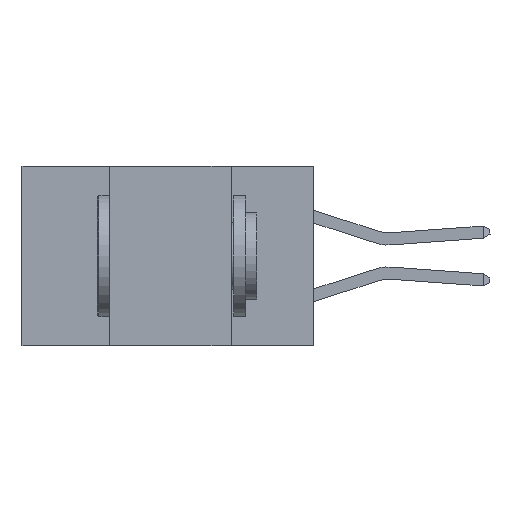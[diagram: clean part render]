
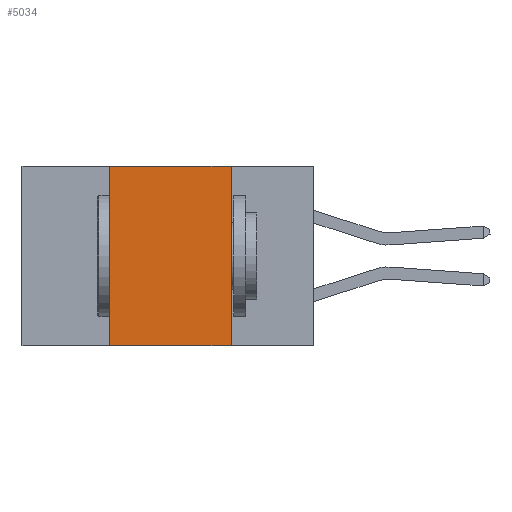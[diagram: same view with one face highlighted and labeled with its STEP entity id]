
A CAD part, left-side view. The second image highlights one B-rep face of the part: STEP entity #5034.
In plain terms, the highlighted planar face has unit normal (-1, 0, 0).
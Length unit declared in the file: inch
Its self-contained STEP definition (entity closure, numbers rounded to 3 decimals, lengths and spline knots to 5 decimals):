
#1138 = CARTESIAN_POINT ( 'NONE',  ( 0., 0.6, -0.37 ) ) ;
#3167 = VECTOR ( 'NONE', #13294, 39.37008 ) ;
#3473 = DIRECTION ( 'NONE',  ( 0., 0., -1. ) ) ;
#4010 = FACE_OUTER_BOUND ( 'NONE', #34146, .T. ) ;
#5034 = ADVANCED_FACE ( 'NONE', ( #4010 ), #29810, .F. ) ;
#6019 = ORIENTED_EDGE ( 'NONE', *, *, #39472, .F. ) ;
#6518 = AXIS2_PLACEMENT_3D ( 'NONE', #7168, #36558, #3473 ) ;
#7168 = CARTESIAN_POINT ( 'NONE',  ( 0., 0.6, 0. ) ) ;
#8007 = CARTESIAN_POINT ( 'NONE',  ( 0., 0.42, 0. ) ) ;
#8116 = VERTEX_POINT ( 'NONE', #30020 ) ;
#9017 = LINE ( 'NONE', #1138, #24797 ) ;
#9627 = LINE ( 'NONE', #25424, #29966 ) ;
#12751 = EDGE_CURVE ( 'NONE', #40426, #8116, #9017, .T. ) ;
#13294 = DIRECTION ( 'NONE',  ( 0., 0., -1. ) ) ;
#13712 = DIRECTION ( 'NONE',  ( 0., -1., 0. ) ) ;
#14030 = CARTESIAN_POINT ( 'NONE',  ( 0., 0.42, -0.37 ) ) ;
#14700 = EDGE_CURVE ( 'NONE', #40426, #26995, #36577, .T. ) ;
#17215 = VECTOR ( 'NONE', #24642, 39.37008 ) ;
#22458 = CARTESIAN_POINT ( 'NONE',  ( 0., 0.17, 0. ) ) ;
#24642 = DIRECTION ( 'NONE',  ( 0., 0., 1. ) ) ;
#24797 = VECTOR ( 'NONE', #13712, 39.37008 ) ;
#25424 = CARTESIAN_POINT ( 'NONE',  ( 0., 0.6, 0. ) ) ;
#26349 = VERTEX_POINT ( 'NONE', #22458 ) ;
#26995 = VERTEX_POINT ( 'NONE', #8007 ) ;
#28503 = ORIENTED_EDGE ( 'NONE', *, *, #12751, .T. ) ;
#29810 = PLANE ( 'NONE',  #6518 ) ;
#29966 = VECTOR ( 'NONE', #32271, 39.37008 ) ;
#30020 = CARTESIAN_POINT ( 'NONE',  ( 0., 0.17, -0.37 ) ) ;
#31458 = EDGE_CURVE ( 'NONE', #26995, #26349, #9627, .T. ) ;
#31617 = LINE ( 'NONE', #35983, #3167 ) ;
#31673 = ORIENTED_EDGE ( 'NONE', *, *, #14700, .F. ) ;
#32271 = DIRECTION ( 'NONE',  ( 0., -1., 0. ) ) ;
#34146 = EDGE_LOOP ( 'NONE', ( #6019, #35402, #31673, #28503 ) ) ;
#35402 = ORIENTED_EDGE ( 'NONE', *, *, #31458, .F. ) ;
#35983 = CARTESIAN_POINT ( 'NONE',  ( 0., 0.17, 0. ) ) ;
#36558 = DIRECTION ( 'NONE',  ( 1., 0., 0. ) ) ;
#36577 = LINE ( 'NONE', #39959, #17215 ) ;
#39472 = EDGE_CURVE ( 'NONE', #26349, #8116, #31617, .T. ) ;
#39959 = CARTESIAN_POINT ( 'NONE',  ( 0., 0.42, 0. ) ) ;
#40426 = VERTEX_POINT ( 'NONE', #14030 ) ;
